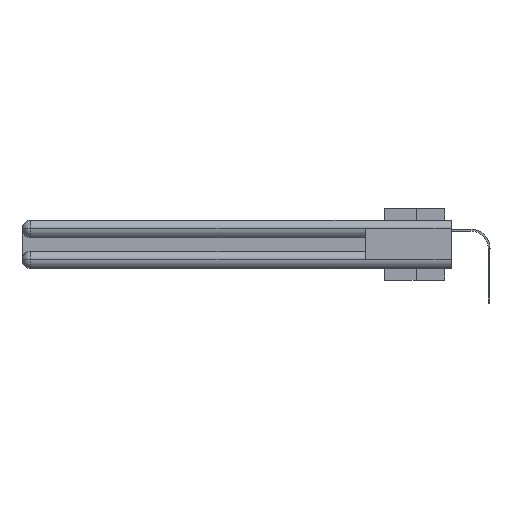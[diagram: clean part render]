
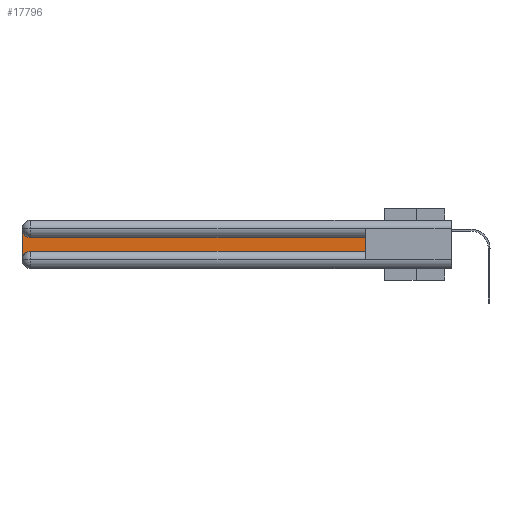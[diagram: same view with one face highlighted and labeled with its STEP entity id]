
A CAD part, left-side view. The second image highlights one B-rep face of the part: STEP entity #17796.
In plain terms, the highlighted planar face has unit normal (-1, 0, 0).
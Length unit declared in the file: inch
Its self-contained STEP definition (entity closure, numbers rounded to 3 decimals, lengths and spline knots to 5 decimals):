
#74 = VERTEX_POINT ( 'NONE', #7072 ) ;
#537 = DIRECTION ( 'NONE',  ( 0., 0., -1. ) ) ;
#617 = EDGE_CURVE ( 'NONE', #74, #17092, #16142, .T. ) ;
#709 = DIRECTION ( 'NONE',  ( 0., 1., 0. ) ) ;
#1111 = DIRECTION ( 'NONE',  ( 0., 0., -1. ) ) ;
#2223 = ORIENTED_EDGE ( 'NONE', *, *, #6208, .T. ) ;
#3134 = DIRECTION ( 'NONE',  ( 0., 0., -1. ) ) ;
#3193 = EDGE_CURVE ( 'NONE', #4876, #11582, #20106, .T. ) ;
#3201 = CARTESIAN_POINT ( 'NONE',  ( 0.075, 3., -0.2175 ) ) ;
#3364 = ORIENTED_EDGE ( 'NONE', *, *, #3193, .T. ) ;
#3419 = AXIS2_PLACEMENT_3D ( 'NONE', #12193, #19274, #1111 ) ;
#3997 = CARTESIAN_POINT ( 'NONE',  ( 0.075, 0.6, -0.2175 ) ) ;
#4084 = VECTOR ( 'NONE', #24810, 39.37008 ) ;
#4876 = VERTEX_POINT ( 'NONE', #16822 ) ;
#4933 = EDGE_CURVE ( 'NONE', #17092, #9782, #25854, .T. ) ;
#5353 = CARTESIAN_POINT ( 'NONE',  ( 0.075, 2.94, -0.0625 ) ) ;
#5570 = CARTESIAN_POINT ( 'NONE',  ( 0.075, 3., -0.1225 ) ) ;
#6153 = VECTOR ( 'NONE', #537, 39.37008 ) ;
#6208 = EDGE_CURVE ( 'NONE', #11582, #74, #14276, .T. ) ;
#7072 = CARTESIAN_POINT ( 'NONE',  ( 0.075, 3., -0.2775 ) ) ;
#7673 = DIRECTION ( 'NONE',  ( 1., 0., 0. ) ) ;
#8099 = FACE_OUTER_BOUND ( 'NONE', #17972, .T. ) ;
#8259 = DIRECTION ( 'NONE',  ( 0., 0., -1. ) ) ;
#9782 = VERTEX_POINT ( 'NONE', #12099 ) ;
#10100 = DIRECTION ( 'NONE',  ( 1., 0., 0. ) ) ;
#10340 = DIRECTION ( 'NONE',  ( 0., -1., 0. ) ) ;
#11582 = VERTEX_POINT ( 'NONE', #22828 ) ;
#12099 = CARTESIAN_POINT ( 'NONE',  ( 0.075, 0.6, -0.2175 ) ) ;
#12193 = CARTESIAN_POINT ( 'NONE',  ( 0.075, 2.94, -0.2775 ) ) ;
#13049 = AXIS2_PLACEMENT_3D ( 'NONE', #5570, #7673, #8259 ) ;
#14276 = LINE ( 'NONE', #3201, #6153 ) ;
#15370 = AXIS2_PLACEMENT_3D ( 'NONE', #5353, #10100, #3134 ) ;
#15375 = CARTESIAN_POINT ( 'NONE',  ( 0.075, 2.94, -0.2175 ) ) ;
#15783 = LINE ( 'NONE', #3997, #4084 ) ;
#16142 = CIRCLE ( 'NONE', #3419, 0.06 ) ;
#16504 = LINE ( 'NONE', #16796, #17006 ) ;
#16796 = CARTESIAN_POINT ( 'NONE',  ( 0.075, 0.6, -0.1225 ) ) ;
#16822 = CARTESIAN_POINT ( 'NONE',  ( 0.075, 2.94, -0.1225 ) ) ;
#17006 = VECTOR ( 'NONE', #709, 39.37008 ) ;
#17092 = VERTEX_POINT ( 'NONE', #15375 ) ;
#17122 = CARTESIAN_POINT ( 'NONE',  ( 0.075, 0.6, -0.2175 ) ) ;
#17367 = ORIENTED_EDGE ( 'NONE', *, *, #617, .T. ) ;
#17435 = EDGE_CURVE ( 'NONE', #9782, #23368, #15783, .T. ) ;
#17796 = ADVANCED_FACE ( 'NONE', ( #8099 ), #23460, .F. ) ;
#17972 = EDGE_LOOP ( 'NONE', ( #19699, #3364, #2223, #17367, #18715, #19763 ) ) ;
#18715 = ORIENTED_EDGE ( 'NONE', *, *, #4933, .T. ) ;
#19274 = DIRECTION ( 'NONE',  ( 1., 0., 0. ) ) ;
#19699 = ORIENTED_EDGE ( 'NONE', *, *, #23492, .T. ) ;
#19763 = ORIENTED_EDGE ( 'NONE', *, *, #17435, .T. ) ;
#20106 = CIRCLE ( 'NONE', #15370, 0.06 ) ;
#22132 = CARTESIAN_POINT ( 'NONE',  ( 0.075, 0.6, -0.1225 ) ) ;
#22828 = CARTESIAN_POINT ( 'NONE',  ( 0.075, 3., -0.0625 ) ) ;
#23368 = VERTEX_POINT ( 'NONE', #22132 ) ;
#23460 = PLANE ( 'NONE',  #13049 ) ;
#23492 = EDGE_CURVE ( 'NONE', #23368, #4876, #16504, .T. ) ;
#24810 = DIRECTION ( 'NONE',  ( 0., 0., 1. ) ) ;
#25854 = LINE ( 'NONE', #17122, #26327 ) ;
#26327 = VECTOR ( 'NONE', #10340, 39.37008 ) ;
